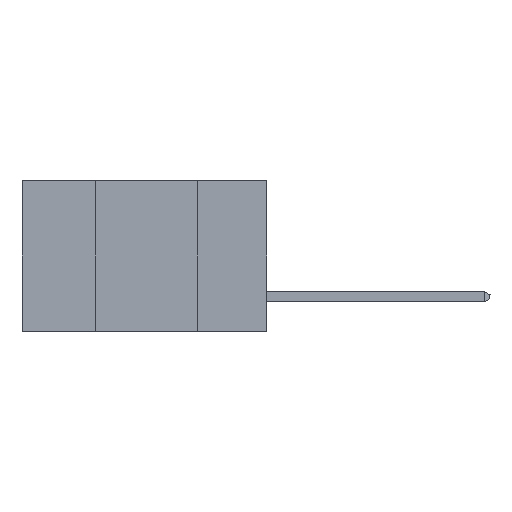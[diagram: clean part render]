
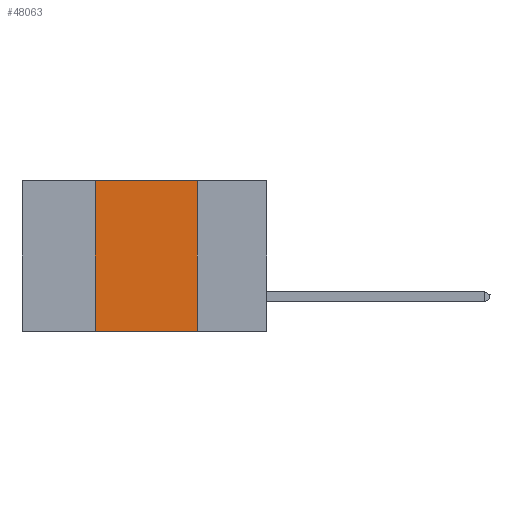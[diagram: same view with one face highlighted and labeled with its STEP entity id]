
A CAD part, left-side view. The second image highlights one B-rep face of the part: STEP entity #48063.
In plain terms, the highlighted planar face has unit normal (-1, 0, 0).
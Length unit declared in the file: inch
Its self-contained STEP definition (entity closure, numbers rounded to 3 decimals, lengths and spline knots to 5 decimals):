
#370 = CARTESIAN_POINT ( 'NONE',  ( 0., 0.42, -0.37 ) ) ;
#619 = EDGE_CURVE ( 'NONE', #40409, #31045, #44711, .T. ) ;
#704 = EDGE_LOOP ( 'NONE', ( #19696, #18215, #17270, #17483 ) ) ;
#833 = VERTEX_POINT ( 'NONE', #47104 ) ;
#857 = EDGE_CURVE ( 'NONE', #40409, #32720, #17096, .T. ) ;
#6344 = CARTESIAN_POINT ( 'NONE',  ( 0., 0.42, 0. ) ) ;
#6651 = DIRECTION ( 'NONE',  ( 0., 0., -1. ) ) ;
#7271 = EDGE_CURVE ( 'NONE', #833, #31045, #14082, .T. ) ;
#10546 = VECTOR ( 'NONE', #29589, 39.37008 ) ;
#10556 = PLANE ( 'NONE',  #19970 ) ;
#11366 = EDGE_CURVE ( 'NONE', #32720, #833, #30296, .T. ) ;
#12462 = CARTESIAN_POINT ( 'NONE',  ( 0., 0.6, 0. ) ) ;
#14082 = LINE ( 'NONE', #33117, #33413 ) ;
#14230 = CARTESIAN_POINT ( 'NONE',  ( 0., 0.6, 0. ) ) ;
#14723 = FACE_OUTER_BOUND ( 'NONE', #704, .T. ) ;
#15189 = CARTESIAN_POINT ( 'NONE',  ( 0., 0.6, -0.37 ) ) ;
#15287 = CARTESIAN_POINT ( 'NONE',  ( 0., 0.42, 0. ) ) ;
#17096 = LINE ( 'NONE', #6344, #48021 ) ;
#17270 = ORIENTED_EDGE ( 'NONE', *, *, #857, .F. ) ;
#17483 = ORIENTED_EDGE ( 'NONE', *, *, #619, .T. ) ;
#18215 = ORIENTED_EDGE ( 'NONE', *, *, #11366, .F. ) ;
#19696 = ORIENTED_EDGE ( 'NONE', *, *, #7271, .F. ) ;
#19787 = DIRECTION ( 'NONE',  ( 0., -1., 0. ) ) ;
#19970 = AXIS2_PLACEMENT_3D ( 'NONE', #14230, #22264, #6651 ) ;
#22264 = DIRECTION ( 'NONE',  ( 1., 0., 0. ) ) ;
#29003 = VECTOR ( 'NONE', #19787, 39.37008 ) ;
#29589 = DIRECTION ( 'NONE',  ( 0., -1., 0. ) ) ;
#30296 = LINE ( 'NONE', #12462, #29003 ) ;
#30694 = CARTESIAN_POINT ( 'NONE',  ( 0., 0.17, -0.37 ) ) ;
#31045 = VERTEX_POINT ( 'NONE', #30694 ) ;
#32720 = VERTEX_POINT ( 'NONE', #15287 ) ;
#33117 = CARTESIAN_POINT ( 'NONE',  ( 0., 0.17, 0. ) ) ;
#33413 = VECTOR ( 'NONE', #40187, 39.37008 ) ;
#35148 = DIRECTION ( 'NONE',  ( 0., 0., 1. ) ) ;
#40187 = DIRECTION ( 'NONE',  ( 0., 0., -1. ) ) ;
#40409 = VERTEX_POINT ( 'NONE', #370 ) ;
#44711 = LINE ( 'NONE', #15189, #10546 ) ;
#47104 = CARTESIAN_POINT ( 'NONE',  ( 0., 0.17, 0. ) ) ;
#48021 = VECTOR ( 'NONE', #35148, 39.37008 ) ;
#48063 = ADVANCED_FACE ( 'NONE', ( #14723 ), #10556, .F. ) ;
